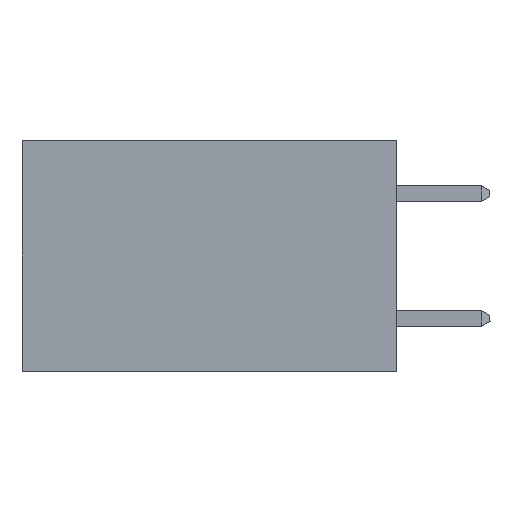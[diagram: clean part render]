
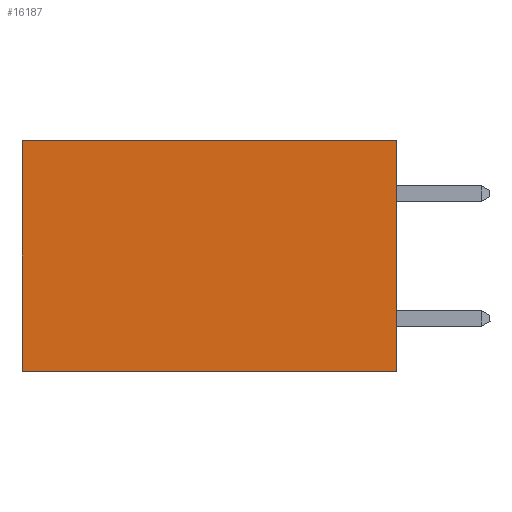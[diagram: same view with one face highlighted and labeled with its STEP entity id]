
A CAD part, left-side view. The second image highlights one B-rep face of the part: STEP entity #16187.
In plain terms, the highlighted planar face has unit normal (-1, 0, 0).
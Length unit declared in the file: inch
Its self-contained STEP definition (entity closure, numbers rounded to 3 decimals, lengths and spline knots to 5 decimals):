
#1354 = ORIENTED_EDGE ( 'NONE', *, *, #22071, .F. ) ;
#2182 = VECTOR ( 'NONE', #9283, 39.37008 ) ;
#2876 = ORIENTED_EDGE ( 'NONE', *, *, #18161, .F. ) ;
#2898 = VERTEX_POINT ( 'NONE', #14837 ) ;
#3493 = DIRECTION ( 'NONE',  ( 0., 1., 0. ) ) ;
#3697 = ORIENTED_EDGE ( 'NONE', *, *, #11017, .T. ) ;
#3727 = CARTESIAN_POINT ( 'NONE',  ( 0.298, 0., 0. ) ) ;
#4671 = CARTESIAN_POINT ( 'NONE',  ( 0.298, 0., 0. ) ) ;
#7120 = LINE ( 'NONE', #7503, #21555 ) ;
#7503 = CARTESIAN_POINT ( 'NONE',  ( 0.298, 0., 0. ) ) ;
#7678 = DIRECTION ( 'NONE',  ( 0., 0., -1. ) ) ;
#9283 = DIRECTION ( 'NONE',  ( 0., 0., -1. ) ) ;
#9320 = VERTEX_POINT ( 'NONE', #11881 ) ;
#9527 = PLANE ( 'NONE',  #14444 ) ;
#9667 = LINE ( 'NONE', #11201, #24013 ) ;
#10301 = CARTESIAN_POINT ( 'NONE',  ( 0.298, 0., 0. ) ) ;
#11017 = EDGE_CURVE ( 'NONE', #19732, #2898, #7120, .T. ) ;
#11201 = CARTESIAN_POINT ( 'NONE',  ( 0.298, 0., -0.37 ) ) ;
#11881 = CARTESIAN_POINT ( 'NONE',  ( 0.298, 0., -0.37 ) ) ;
#12351 = VERTEX_POINT ( 'NONE', #22493 ) ;
#14137 = EDGE_LOOP ( 'NONE', ( #21401, #2876, #1354, #3697 ) ) ;
#14444 = AXIS2_PLACEMENT_3D ( 'NONE', #3727, #18951, #7678 ) ;
#14837 = CARTESIAN_POINT ( 'NONE',  ( 0.298, 0.6, 0. ) ) ;
#15328 = VECTOR ( 'NONE', #21778, 39.37008 ) ;
#15909 = LINE ( 'NONE', #4671, #15328 ) ;
#16187 = ADVANCED_FACE ( 'NONE', ( #24384 ), #9527, .F. ) ;
#16612 = EDGE_CURVE ( 'NONE', #2898, #12351, #22960, .T. ) ;
#18161 = EDGE_CURVE ( 'NONE', #9320, #12351, #9667, .T. ) ;
#18951 = DIRECTION ( 'NONE',  ( 1., 0., 0. ) ) ;
#19732 = VERTEX_POINT ( 'NONE', #10301 ) ;
#21401 = ORIENTED_EDGE ( 'NONE', *, *, #16612, .T. ) ;
#21555 = VECTOR ( 'NONE', #22549, 39.37008 ) ;
#21778 = DIRECTION ( 'NONE',  ( 0., 0., -1. ) ) ;
#22071 = EDGE_CURVE ( 'NONE', #19732, #9320, #15909, .T. ) ;
#22493 = CARTESIAN_POINT ( 'NONE',  ( 0.298, 0.6, -0.37 ) ) ;
#22549 = DIRECTION ( 'NONE',  ( 0., 1., 0. ) ) ;
#22960 = LINE ( 'NONE', #24236, #2182 ) ;
#24013 = VECTOR ( 'NONE', #3493, 39.37008 ) ;
#24236 = CARTESIAN_POINT ( 'NONE',  ( 0.298, 0.6, 0. ) ) ;
#24384 = FACE_OUTER_BOUND ( 'NONE', #14137, .T. ) ;
